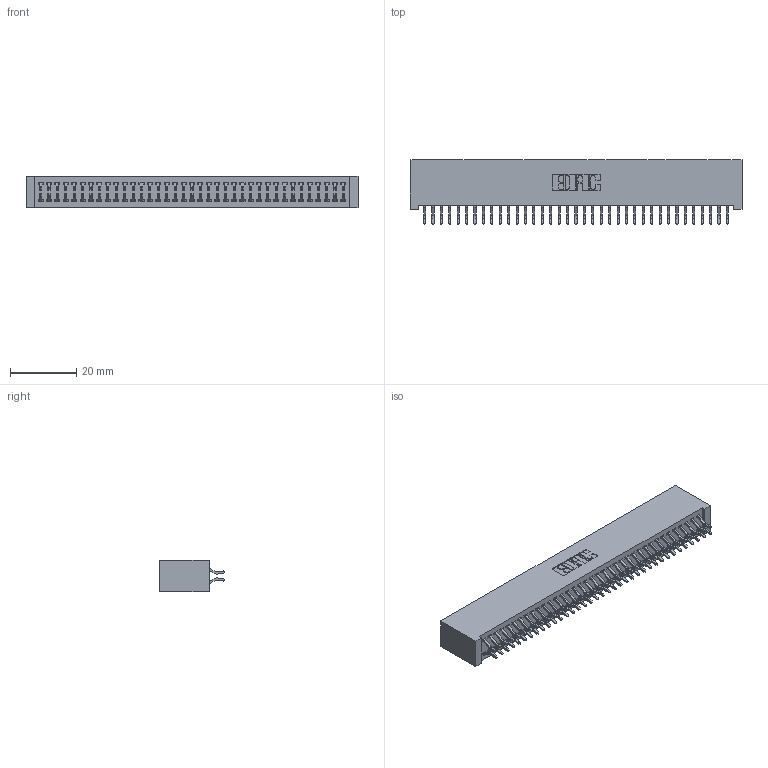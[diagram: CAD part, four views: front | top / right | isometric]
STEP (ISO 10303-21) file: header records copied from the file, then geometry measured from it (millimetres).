
FILE_DESCRIPTION (( 'STEP AP203' ), '1' );
FILE_NAME ('342-074-556-201.STEP', '2018-08-13T11:40:50', ( '' ), ( '' ), 'SwSTEP 2.0', 'SolidWorks 2016', '' );
FILE_SCHEMA (( 'CONFIG_CONTROL_DESIGN' ));
Length unit declared in the file: inch
Products named in the file (3): 342 Part_Lugless; 345-292-001_556 Tail; 342-074-556-201
Assembly tree (75 placements, depth 2):
  342-074-556-201
    342 Part_Lugless
    345-292-001_556 Tail  x74
Bounding box: 100.23 x 19.58 x 9.4 mm (x, y, z)
Volume: 9419.5 mm3; surface area: 15583.8 mm2
Topology: 75 solids, 75 shells, 4394 faces, 13077 edges, 8618 vertices
Faces by surface type: plane 3022, cylinder 1372
Entity records: 24261 total; most frequent: CARTESIAN_POINT 4038, ORIENTED_EDGE 3962, DIRECTION 3441, EDGE_CURVE 1981, VECTOR 1853, LINE 1853, VERTEX_POINT 1318, AXIS2_PLACEMENT_3D 794
